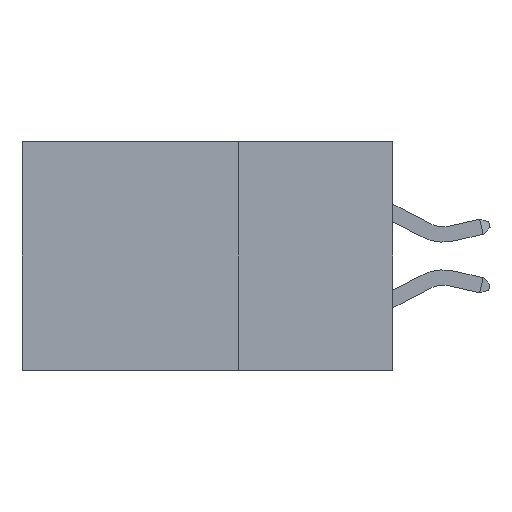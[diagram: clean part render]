
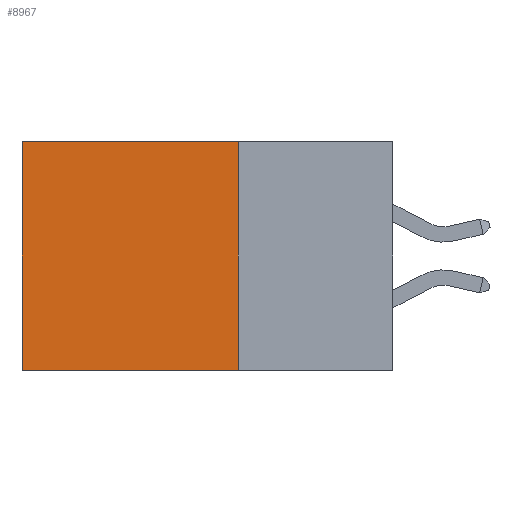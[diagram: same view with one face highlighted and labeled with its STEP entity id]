
A CAD part, left-side view. The second image highlights one B-rep face of the part: STEP entity #8967.
In plain terms, the highlighted planar face has unit normal (-1, 0, 0).
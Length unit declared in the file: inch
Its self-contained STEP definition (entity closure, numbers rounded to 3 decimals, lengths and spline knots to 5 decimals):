
#199 = AXIS2_PLACEMENT_3D ( 'NONE', #2724, #7627, #3455 ) ;
#363 = ORIENTED_EDGE ( 'NONE', *, *, #1459, .F. ) ;
#922 = EDGE_CURVE ( 'NONE', #2125, #2697, #4197, .T. ) ;
#1338 = DIRECTION ( 'NONE',  ( 0., 0., -1. ) ) ;
#1459 = EDGE_CURVE ( 'NONE', #2697, #3101, #3537, .T. ) ;
#1521 = LINE ( 'NONE', #3220, #3298 ) ;
#1600 = ORIENTED_EDGE ( 'NONE', *, *, #922, .F. ) ;
#1970 = VECTOR ( 'NONE', #7839, 39.37008 ) ;
#1989 = EDGE_CURVE ( 'NONE', #2125, #4176, #1521, .T. ) ;
#2125 = VERTEX_POINT ( 'NONE', #8204 ) ;
#2697 = VERTEX_POINT ( 'NONE', #7287 ) ;
#2724 = CARTESIAN_POINT ( 'NONE',  ( 0.2875, 0.25, 0. ) ) ;
#3101 = VERTEX_POINT ( 'NONE', #7262 ) ;
#3220 = CARTESIAN_POINT ( 'NONE',  ( 0.2875, 0.25, 0. ) ) ;
#3281 = EDGE_LOOP ( 'NONE', ( #4553, #363, #1600, #4836 ) ) ;
#3298 = VECTOR ( 'NONE', #8146, 39.37008 ) ;
#3311 = VECTOR ( 'NONE', #9069, 39.37008 ) ;
#3455 = DIRECTION ( 'NONE',  ( 0., 0., -1. ) ) ;
#3537 = LINE ( 'NONE', #8984, #3311 ) ;
#3902 = LINE ( 'NONE', #5780, #1970 ) ;
#3958 = VECTOR ( 'NONE', #1338, 39.37008 ) ;
#4176 = VERTEX_POINT ( 'NONE', #7700 ) ;
#4197 = LINE ( 'NONE', #7323, #3958 ) ;
#4553 = ORIENTED_EDGE ( 'NONE', *, *, #7971, .T. ) ;
#4817 = PLANE ( 'NONE',  #199 ) ;
#4836 = ORIENTED_EDGE ( 'NONE', *, *, #1989, .T. ) ;
#5780 = CARTESIAN_POINT ( 'NONE',  ( 0.2875, 0.6, 0. ) ) ;
#7262 = CARTESIAN_POINT ( 'NONE',  ( 0.2875, 0.6, -0.37 ) ) ;
#7287 = CARTESIAN_POINT ( 'NONE',  ( 0.2875, 0.25, -0.37 ) ) ;
#7323 = CARTESIAN_POINT ( 'NONE',  ( 0.2875, 0.25, 0. ) ) ;
#7627 = DIRECTION ( 'NONE',  ( 1., 0., 0. ) ) ;
#7700 = CARTESIAN_POINT ( 'NONE',  ( 0.2875, 0.6, 0. ) ) ;
#7703 = FACE_OUTER_BOUND ( 'NONE', #3281, .T. ) ;
#7839 = DIRECTION ( 'NONE',  ( 0., 0., -1. ) ) ;
#7971 = EDGE_CURVE ( 'NONE', #4176, #3101, #3902, .T. ) ;
#8146 = DIRECTION ( 'NONE',  ( 0., 1., 0. ) ) ;
#8204 = CARTESIAN_POINT ( 'NONE',  ( 0.2875, 0.25, 0. ) ) ;
#8967 = ADVANCED_FACE ( 'NONE', ( #7703 ), #4817, .F. ) ;
#8984 = CARTESIAN_POINT ( 'NONE',  ( 0.2875, 0.25, -0.37 ) ) ;
#9069 = DIRECTION ( 'NONE',  ( 0., 1., 0. ) ) ;
